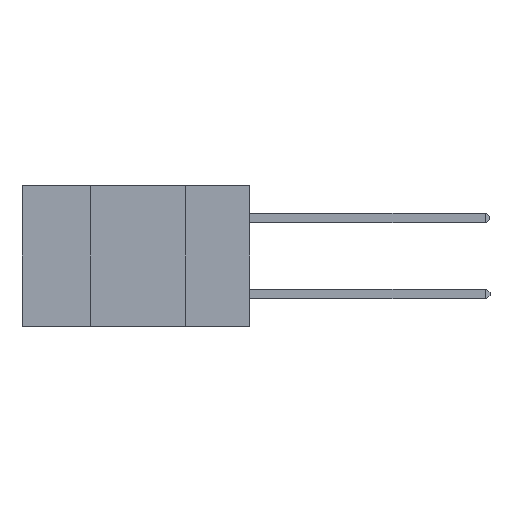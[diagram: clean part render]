
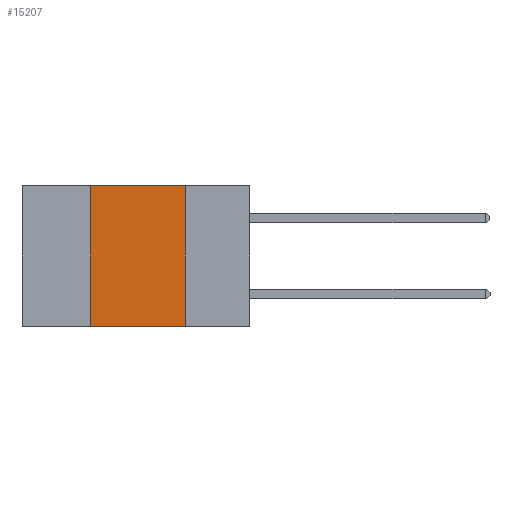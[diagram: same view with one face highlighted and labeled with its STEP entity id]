
A CAD part, left-side view. The second image highlights one B-rep face of the part: STEP entity #15207.
In plain terms, the highlighted planar face has unit normal (-1, 0, 0).
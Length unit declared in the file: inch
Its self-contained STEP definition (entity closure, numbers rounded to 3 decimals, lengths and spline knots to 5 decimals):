
#833 = DIRECTION ( 'NONE',  ( 0., 0., -1. ) ) ;
#1192 = CARTESIAN_POINT ( 'NONE',  ( 0., 0.17, -0.37 ) ) ;
#1582 = VERTEX_POINT ( 'NONE', #2260 ) ;
#1920 = PLANE ( 'NONE',  #10501 ) ;
#2260 = CARTESIAN_POINT ( 'NONE',  ( 0., 0.42, 0. ) ) ;
#2454 = VECTOR ( 'NONE', #22030, 39.37008 ) ;
#3708 = VECTOR ( 'NONE', #12413, 39.37008 ) ;
#6265 = EDGE_LOOP ( 'NONE', ( #17791, #19205, #8198, #17934 ) ) ;
#6461 = DIRECTION ( 'NONE',  ( 0., 0., 1. ) ) ;
#7460 = DIRECTION ( 'NONE',  ( 0., -1., 0. ) ) ;
#8198 = ORIENTED_EDGE ( 'NONE', *, *, #13092, .F. ) ;
#9491 = CARTESIAN_POINT ( 'NONE',  ( 0., 0.42, -0.37 ) ) ;
#9592 = VECTOR ( 'NONE', #7460, 39.37008 ) ;
#10501 = AXIS2_PLACEMENT_3D ( 'NONE', #23292, #15918, #833 ) ;
#10857 = FACE_OUTER_BOUND ( 'NONE', #6265, .T. ) ;
#10917 = EDGE_CURVE ( 'NONE', #16732, #19672, #14538, .T. ) ;
#12413 = DIRECTION ( 'NONE',  ( 0., -1., 0. ) ) ;
#13092 = EDGE_CURVE ( 'NONE', #16732, #1582, #19059, .T. ) ;
#13243 = CARTESIAN_POINT ( 'NONE',  ( 0., 0.6, 0. ) ) ;
#14538 = LINE ( 'NONE', #23381, #9592 ) ;
#15207 = ADVANCED_FACE ( 'NONE', ( #10857 ), #1920, .F. ) ;
#15546 = LINE ( 'NONE', #16514, #2454 ) ;
#15636 = CARTESIAN_POINT ( 'NONE',  ( 0., 0.42, 0. ) ) ;
#15918 = DIRECTION ( 'NONE',  ( 1., 0., 0. ) ) ;
#16514 = CARTESIAN_POINT ( 'NONE',  ( 0., 0.17, 0. ) ) ;
#16732 = VERTEX_POINT ( 'NONE', #9491 ) ;
#17791 = ORIENTED_EDGE ( 'NONE', *, *, #23229, .F. ) ;
#17873 = EDGE_CURVE ( 'NONE', #1582, #20769, #23753, .T. ) ;
#17934 = ORIENTED_EDGE ( 'NONE', *, *, #10917, .T. ) ;
#19059 = LINE ( 'NONE', #15636, #21924 ) ;
#19205 = ORIENTED_EDGE ( 'NONE', *, *, #17873, .F. ) ;
#19672 = VERTEX_POINT ( 'NONE', #1192 ) ;
#20769 = VERTEX_POINT ( 'NONE', #21424 ) ;
#21424 = CARTESIAN_POINT ( 'NONE',  ( 0., 0.17, 0. ) ) ;
#21924 = VECTOR ( 'NONE', #6461, 39.37008 ) ;
#22030 = DIRECTION ( 'NONE',  ( 0., 0., -1. ) ) ;
#23229 = EDGE_CURVE ( 'NONE', #20769, #19672, #15546, .T. ) ;
#23292 = CARTESIAN_POINT ( 'NONE',  ( 0., 0.6, 0. ) ) ;
#23381 = CARTESIAN_POINT ( 'NONE',  ( 0., 0.6, -0.37 ) ) ;
#23753 = LINE ( 'NONE', #13243, #3708 ) ;
